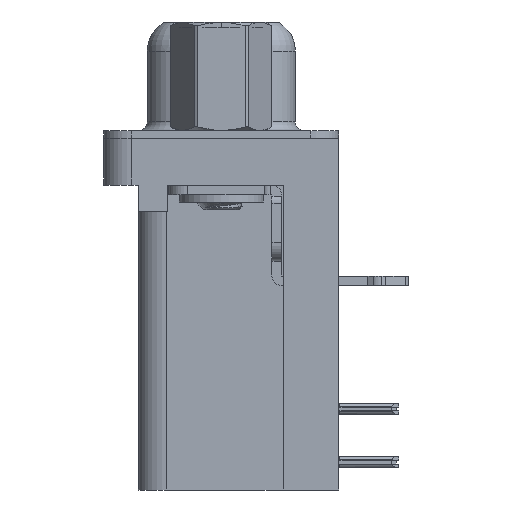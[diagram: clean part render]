
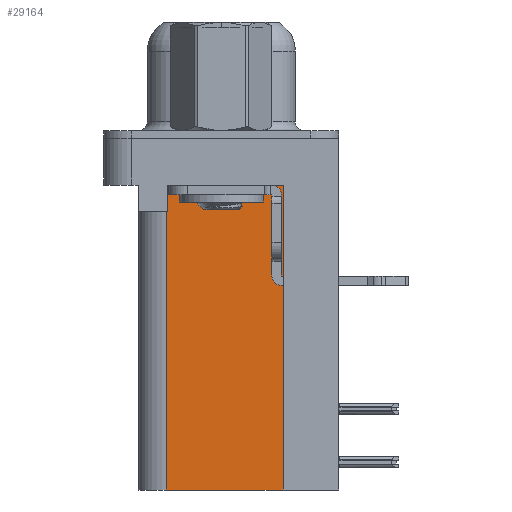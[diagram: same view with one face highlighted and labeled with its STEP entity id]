
A CAD part, left-side view. The second image highlights one B-rep face of the part: STEP entity #29164.
In plain terms, the highlighted planar face has unit normal (-1, 0, 0).
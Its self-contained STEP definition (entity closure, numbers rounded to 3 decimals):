
#2268 = VERTEX_POINT ( 'NONE', #22341 ) ;
#2380 = EDGE_CURVE ( 'NONE', #26023, #12216, #33526, .T. ) ;
#2977 = DIRECTION ( 'NONE',  ( 0., 1., 0. ) ) ;
#3564 = CARTESIAN_POINT ( 'NONE',  ( 3.79, -3.295, -18.76 ) ) ;
#4084 = DIRECTION ( 'NONE',  ( 0., 0., -1. ) ) ;
#4260 = CARTESIAN_POINT ( 'NONE',  ( 3.79, 2.925, -18.76 ) ) ;
#6436 = VECTOR ( 'NONE', #7643, 1000. ) ;
#6475 = LINE ( 'NONE', #4260, #6436 ) ;
#6923 = DIRECTION ( 'NONE',  ( 0., 0., 1. ) ) ;
#7430 = EDGE_CURVE ( 'NONE', #32780, #2268, #39700, .T. ) ;
#7643 = DIRECTION ( 'NONE',  ( 0., 0., 1. ) ) ;
#7829 = EDGE_CURVE ( 'NONE', #32780, #26023, #36425, .T. ) ;
#8634 = EDGE_CURVE ( 'NONE', #12216, #17223, #29353, .T. ) ;
#10406 = ORIENTED_EDGE ( 'NONE', *, *, #40685, .F. ) ;
#10830 = CARTESIAN_POINT ( 'NONE',  ( 3.79, 2.895, -3.9 ) ) ;
#12128 = EDGE_CURVE ( 'NONE', #17223, #37451, #22518, .T. ) ;
#12216 = VERTEX_POINT ( 'NONE', #27689 ) ;
#16405 = PLANE ( 'NONE',  #26479 ) ;
#16888 = ORIENTED_EDGE ( 'NONE', *, *, #2380, .T. ) ;
#17223 = VERTEX_POINT ( 'NONE', #10830 ) ;
#17830 = DIRECTION ( 'NONE',  ( 0., 1., 0. ) ) ;
#18575 = ORIENTED_EDGE ( 'NONE', *, *, #7430, .F. ) ;
#19707 = CARTESIAN_POINT ( 'NONE',  ( 3.79, -3.295, -18.76 ) ) ;
#21158 = CARTESIAN_POINT ( 'NONE',  ( 3.79, 2.925, -3.9 ) ) ;
#22341 = CARTESIAN_POINT ( 'NONE',  ( 3.79, 2.925, -18.76 ) ) ;
#22518 = LINE ( 'NONE', #37004, #28470 ) ;
#23014 = DIRECTION ( 'NONE',  ( 1., 0., 0. ) ) ;
#23745 = ORIENTED_EDGE ( 'NONE', *, *, #7829, .T. ) ;
#26023 = VERTEX_POINT ( 'NONE', #28410 ) ;
#26479 = AXIS2_PLACEMENT_3D ( 'NONE', #19707, #23014, #2977 ) ;
#26700 = CARTESIAN_POINT ( 'NONE',  ( 3.79, -3.295, -18.76 ) ) ;
#26804 = ORIENTED_EDGE ( 'NONE', *, *, #12128, .T. ) ;
#27138 = CARTESIAN_POINT ( 'NONE',  ( 3.79, 2.895, -3.9 ) ) ;
#27689 = CARTESIAN_POINT ( 'NONE',  ( 3.79, 2.895, -2.5 ) ) ;
#28410 = CARTESIAN_POINT ( 'NONE',  ( 3.79, -3.295, -2.5 ) ) ;
#28470 = VECTOR ( 'NONE', #40099, 1000. ) ;
#28815 = VECTOR ( 'NONE', #4084, 1000. ) ;
#29164 = ADVANCED_FACE ( 'NONE', ( #40885 ), #16405, .F. ) ;
#29353 = LINE ( 'NONE', #27138, #28815 ) ;
#30921 = DIRECTION ( 'NONE',  ( 0., 1., 0. ) ) ;
#31355 = CARTESIAN_POINT ( 'NONE',  ( 3.79, -3.295, -2.5 ) ) ;
#32780 = VERTEX_POINT ( 'NONE', #26700 ) ;
#33093 = EDGE_LOOP ( 'NONE', ( #16888, #33838, #26804, #10406, #18575, #23745 ) ) ;
#33372 = VECTOR ( 'NONE', #30921, 1000. ) ;
#33526 = LINE ( 'NONE', #31355, #33372 ) ;
#33682 = CARTESIAN_POINT ( 'NONE',  ( 3.79, -3.295, -18.76 ) ) ;
#33838 = ORIENTED_EDGE ( 'NONE', *, *, #8634, .T. ) ;
#36335 = VECTOR ( 'NONE', #6923, 1000. ) ;
#36425 = LINE ( 'NONE', #3564, #36335 ) ;
#37004 = CARTESIAN_POINT ( 'NONE',  ( 3.79, 0., -3.9 ) ) ;
#37451 = VERTEX_POINT ( 'NONE', #21158 ) ;
#39659 = VECTOR ( 'NONE', #17830, 1000. ) ;
#39700 = LINE ( 'NONE', #33682, #39659 ) ;
#40099 = DIRECTION ( 'NONE',  ( 0., 1., 0. ) ) ;
#40685 = EDGE_CURVE ( 'NONE', #2268, #37451, #6475, .T. ) ;
#40885 = FACE_OUTER_BOUND ( 'NONE', #33093, .T. ) ;
